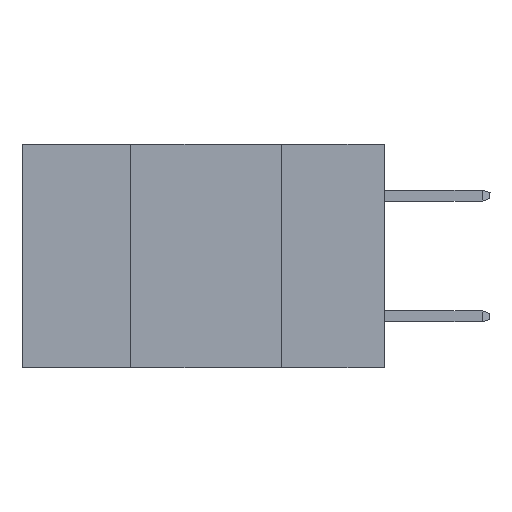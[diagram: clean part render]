
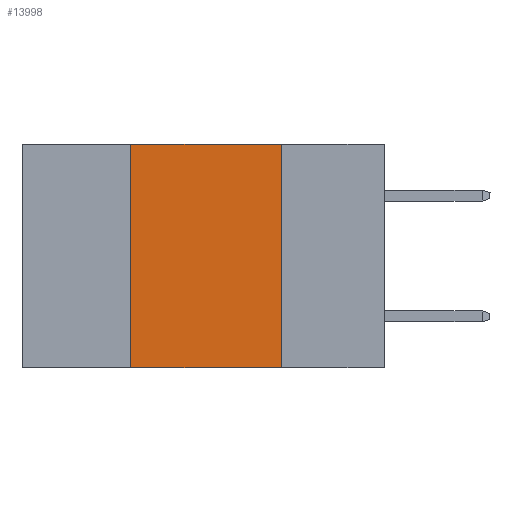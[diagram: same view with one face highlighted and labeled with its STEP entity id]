
A CAD part, left-side view. The second image highlights one B-rep face of the part: STEP entity #13998.
In plain terms, the highlighted planar face has unit normal (-1, 0, 0).
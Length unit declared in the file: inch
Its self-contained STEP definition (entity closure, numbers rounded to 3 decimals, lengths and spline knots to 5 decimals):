
#1084 = VERTEX_POINT ( 'NONE', #22587 ) ;
#1196 = LINE ( 'NONE', #11508, #14759 ) ;
#1492 = CARTESIAN_POINT ( 'NONE',  ( 0., 0.17, -0.37 ) ) ;
#2591 = LINE ( 'NONE', #7847, #19605 ) ;
#2740 = ORIENTED_EDGE ( 'NONE', *, *, #11278, .F. ) ;
#3194 = EDGE_CURVE ( 'NONE', #1084, #20295, #2591, .T. ) ;
#6725 = ORIENTED_EDGE ( 'NONE', *, *, #23102, .F. ) ;
#7382 = ORIENTED_EDGE ( 'NONE', *, *, #9855, .T. ) ;
#7847 = CARTESIAN_POINT ( 'NONE',  ( 0., 0.42, 0. ) ) ;
#8055 = CARTESIAN_POINT ( 'NONE',  ( 0., 0.17, 0. ) ) ;
#8721 = EDGE_LOOP ( 'NONE', ( #6725, #2740, #12619, #7382 ) ) ;
#9662 = VERTEX_POINT ( 'NONE', #1492 ) ;
#9855 = EDGE_CURVE ( 'NONE', #1084, #9662, #23602, .T. ) ;
#11278 = EDGE_CURVE ( 'NONE', #20295, #17899, #1196, .T. ) ;
#11508 = CARTESIAN_POINT ( 'NONE',  ( 0., 0.6, 0. ) ) ;
#12619 = ORIENTED_EDGE ( 'NONE', *, *, #3194, .F. ) ;
#12930 = AXIS2_PLACEMENT_3D ( 'NONE', #25614, #18723, #18824 ) ;
#13207 = DIRECTION ( 'NONE',  ( 0., 0., -1. ) ) ;
#13998 = ADVANCED_FACE ( 'NONE', ( #20912 ), #20893, .F. ) ;
#14348 = CARTESIAN_POINT ( 'NONE',  ( 0., 0.42, 0. ) ) ;
#14759 = VECTOR ( 'NONE', #20041, 39.37008 ) ;
#17703 = CARTESIAN_POINT ( 'NONE',  ( 0., 0.6, -0.37 ) ) ;
#17899 = VERTEX_POINT ( 'NONE', #28539 ) ;
#18558 = LINE ( 'NONE', #8055, #25239 ) ;
#18723 = DIRECTION ( 'NONE',  ( 1., 0., 0. ) ) ;
#18824 = DIRECTION ( 'NONE',  ( 0., 0., -1. ) ) ;
#19605 = VECTOR ( 'NONE', #23702, 39.37008 ) ;
#20041 = DIRECTION ( 'NONE',  ( 0., -1., 0. ) ) ;
#20295 = VERTEX_POINT ( 'NONE', #14348 ) ;
#20893 = PLANE ( 'NONE',  #12930 ) ;
#20912 = FACE_OUTER_BOUND ( 'NONE', #8721, .T. ) ;
#22587 = CARTESIAN_POINT ( 'NONE',  ( 0., 0.42, -0.37 ) ) ;
#23102 = EDGE_CURVE ( 'NONE', #17899, #9662, #18558, .T. ) ;
#23602 = LINE ( 'NONE', #17703, #27469 ) ;
#23702 = DIRECTION ( 'NONE',  ( 0., 0., 1. ) ) ;
#24178 = DIRECTION ( 'NONE',  ( 0., -1., 0. ) ) ;
#25239 = VECTOR ( 'NONE', #13207, 39.37008 ) ;
#25614 = CARTESIAN_POINT ( 'NONE',  ( 0., 0.6, 0. ) ) ;
#27469 = VECTOR ( 'NONE', #24178, 39.37008 ) ;
#28539 = CARTESIAN_POINT ( 'NONE',  ( 0., 0.17, 0. ) ) ;
